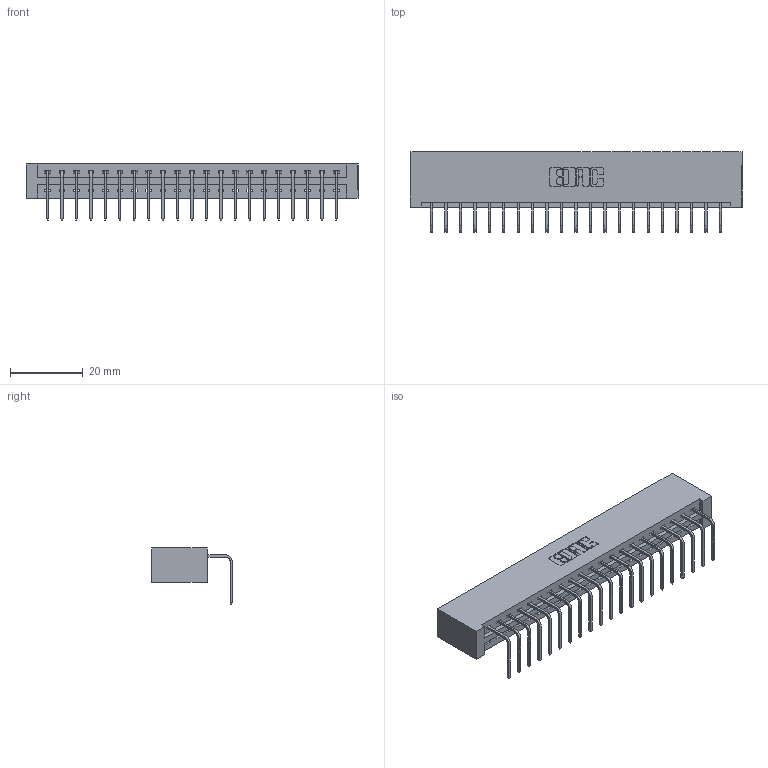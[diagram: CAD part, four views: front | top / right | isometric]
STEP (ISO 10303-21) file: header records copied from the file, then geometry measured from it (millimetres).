
FILE_DESCRIPTION (( 'STEP AP203' ), '1' );
FILE_NAME ('337-021-558-101.STEP', '2018-08-05T12:05:50', ( '' ), ( '' ), 'SwSTEP 2.0', 'SolidWorks 2016', '' );
FILE_SCHEMA (( 'CONFIG_CONTROL_DESIGN' ));
Length unit declared in the file: inch
Products named in the file (3): 337 Part_No Mounting Lugs; 345-292-001_558 Tail - 2; 337-021-558-101
Assembly tree (22 placements, depth 2):
  337-021-558-101
    337 Part_No Mounting Lugs
    345-292-001_558 Tail - 2  x21
Bounding box: 91.08 x 22.17 x 15.37 mm (x, y, z)
Volume: 10012.6 mm3; surface area: 10641.3 mm2
Topology: 22 solids, 22 shells, 1450 faces, 4361 edges, 2878 vertices
Faces by surface type: plane 1074, cylinder 376
Entity records: 18133 total; most frequent: CARTESIAN_POINT 3165, ORIENTED_EDGE 3122, DIRECTION 2699, EDGE_CURVE 1561, VECTOR 1441, LINE 1441, VERTEX_POINT 1038, AXIS2_PLACEMENT_3D 629
